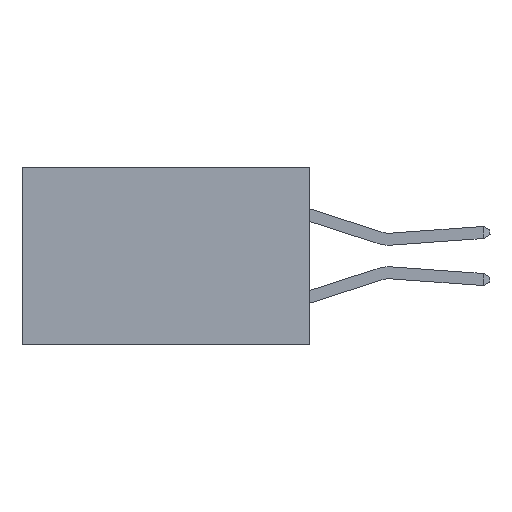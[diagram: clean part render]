
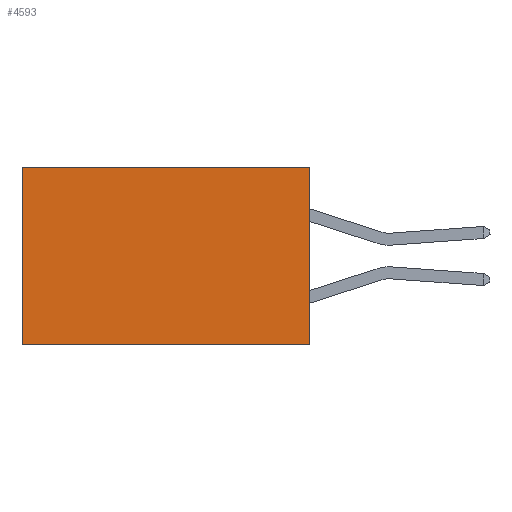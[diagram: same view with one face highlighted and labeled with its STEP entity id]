
A CAD part, left-side view. The second image highlights one B-rep face of the part: STEP entity #4593.
In plain terms, the highlighted planar face has unit normal (-1, 0, 0).
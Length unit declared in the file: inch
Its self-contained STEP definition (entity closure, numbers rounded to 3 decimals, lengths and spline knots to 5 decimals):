
#713 = VERTEX_POINT ( 'NONE', #14767 ) ;
#2069 = CARTESIAN_POINT ( 'NONE',  ( 0.2615, 0., -0.37 ) ) ;
#2491 = VERTEX_POINT ( 'NONE', #6581 ) ;
#2620 = DIRECTION ( 'NONE',  ( 0., 0., -1. ) ) ;
#2624 = DIRECTION ( 'NONE',  ( 0., 1., 0. ) ) ;
#2761 = CARTESIAN_POINT ( 'NONE',  ( 0.2615, 0., 0. ) ) ;
#3274 = VECTOR ( 'NONE', #6209, 39.37008 ) ;
#4593 = ADVANCED_FACE ( 'NONE', ( #8035 ), #12305, .F. ) ;
#5308 = ORIENTED_EDGE ( 'NONE', *, *, #13289, .F. ) ;
#6209 = DIRECTION ( 'NONE',  ( 0., 1., 0. ) ) ;
#6581 = CARTESIAN_POINT ( 'NONE',  ( 0.2615, 0., -0.37 ) ) ;
#7339 = EDGE_CURVE ( 'NONE', #19345, #10682, #12521, .T. ) ;
#8035 = FACE_OUTER_BOUND ( 'NONE', #11091, .T. ) ;
#8660 = CARTESIAN_POINT ( 'NONE',  ( 0.2615, 0.6, -0.37 ) ) ;
#9606 = VECTOR ( 'NONE', #2624, 39.37008 ) ;
#10682 = VERTEX_POINT ( 'NONE', #8660 ) ;
#11091 = EDGE_LOOP ( 'NONE', ( #12372, #15363, #5308, #12295 ) ) ;
#11109 = DIRECTION ( 'NONE',  ( 1., 0., 0. ) ) ;
#12295 = ORIENTED_EDGE ( 'NONE', *, *, #15476, .T. ) ;
#12305 = PLANE ( 'NONE',  #15866 ) ;
#12372 = ORIENTED_EDGE ( 'NONE', *, *, #7339, .T. ) ;
#12521 = LINE ( 'NONE', #18504, #14021 ) ;
#13289 = EDGE_CURVE ( 'NONE', #713, #2491, #14558, .T. ) ;
#13781 = LINE ( 'NONE', #2761, #3274 ) ;
#14021 = VECTOR ( 'NONE', #14415, 39.37008 ) ;
#14108 = DIRECTION ( 'NONE',  ( 0., 0., -1. ) ) ;
#14415 = DIRECTION ( 'NONE',  ( 0., 0., -1. ) ) ;
#14462 = CARTESIAN_POINT ( 'NONE',  ( 0.2615, 0., -0.37 ) ) ;
#14486 = EDGE_CURVE ( 'NONE', #2491, #10682, #17558, .T. ) ;
#14558 = LINE ( 'NONE', #19155, #15970 ) ;
#14767 = CARTESIAN_POINT ( 'NONE',  ( 0.2615, 0., 0. ) ) ;
#15363 = ORIENTED_EDGE ( 'NONE', *, *, #14486, .F. ) ;
#15476 = EDGE_CURVE ( 'NONE', #713, #19345, #13781, .T. ) ;
#15866 = AXIS2_PLACEMENT_3D ( 'NONE', #2069, #11109, #14108 ) ;
#15970 = VECTOR ( 'NONE', #2620, 39.37008 ) ;
#17558 = LINE ( 'NONE', #14462, #9606 ) ;
#18504 = CARTESIAN_POINT ( 'NONE',  ( 0.2615, 0.6, -0.37 ) ) ;
#19091 = CARTESIAN_POINT ( 'NONE',  ( 0.2615, 0.6, 0. ) ) ;
#19155 = CARTESIAN_POINT ( 'NONE',  ( 0.2615, 0., -0.37 ) ) ;
#19345 = VERTEX_POINT ( 'NONE', #19091 ) ;
